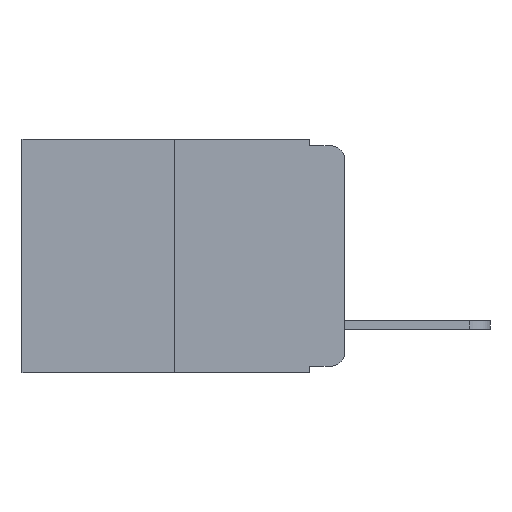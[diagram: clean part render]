
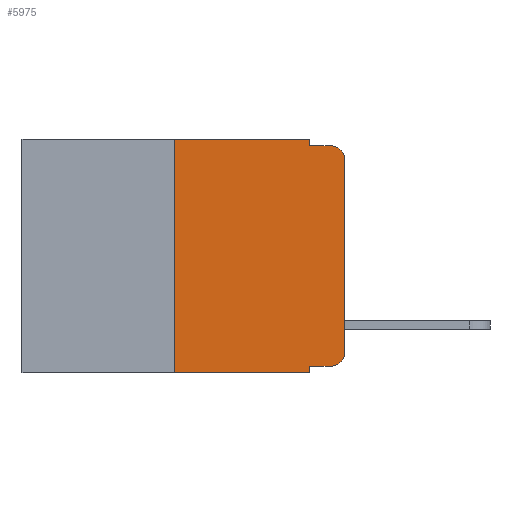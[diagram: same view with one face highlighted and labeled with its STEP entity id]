
A CAD part, left-side view. The second image highlights one B-rep face of the part: STEP entity #5975.
In plain terms, the highlighted planar face has unit normal (-1, 0, 0).
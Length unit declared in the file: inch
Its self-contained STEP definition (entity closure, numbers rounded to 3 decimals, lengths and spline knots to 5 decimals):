
#351 = CARTESIAN_POINT ( 'NONE',  ( 0., 0.473, 0. ) ) ;
#781 = CARTESIAN_POINT ( 'NONE',  ( 0., 0.051, 0. ) ) ;
#1145 = DIRECTION ( 'NONE',  ( 0., 0., -1. ) ) ;
#1237 = ORIENTED_EDGE ( 'NONE', *, *, #7425, .T. ) ;
#1449 = VERTEX_POINT ( 'NONE', #8383 ) ;
#1542 = CARTESIAN_POINT ( 'NONE',  ( 0., 0.02, -0.01 ) ) ;
#1710 = DIRECTION ( 'NONE',  ( 0., -1., 0. ) ) ;
#1713 = VERTEX_POINT ( 'NONE', #12270 ) ;
#1720 = DIRECTION ( 'NONE',  ( 0., 0., 1. ) ) ;
#1800 = FACE_OUTER_BOUND ( 'NONE', #14983, .T. ) ;
#2052 = LINE ( 'NONE', #19518, #5740 ) ;
#2232 = CARTESIAN_POINT ( 'NONE',  ( 0., 0.051, -0.333 ) ) ;
#2244 = EDGE_CURVE ( 'NONE', #5757, #9599, #10545, .T. ) ;
#2960 = VECTOR ( 'NONE', #1720, 39.37008 ) ;
#3056 = AXIS2_PLACEMENT_3D ( 'NONE', #4545, #17236, #6187 ) ;
#3840 = VERTEX_POINT ( 'NONE', #1542 ) ;
#3884 = VERTEX_POINT ( 'NONE', #6210 ) ;
#3897 = DIRECTION ( 'NONE',  ( 0., 0., -1. ) ) ;
#4142 = CARTESIAN_POINT ( 'NONE',  ( 0., 0.25, 0. ) ) ;
#4191 = ORIENTED_EDGE ( 'NONE', *, *, #17792, .F. ) ;
#4386 = ORIENTED_EDGE ( 'NONE', *, *, #19611, .T. ) ;
#4545 = CARTESIAN_POINT ( 'NONE',  ( 0., 0.02, -0.313 ) ) ;
#4651 = EDGE_CURVE ( 'NONE', #17564, #9599, #8992, .T. ) ;
#5457 = VERTEX_POINT ( 'NONE', #11801 ) ;
#5740 = VECTOR ( 'NONE', #13293, 39.37008 ) ;
#5757 = VERTEX_POINT ( 'NONE', #18464 ) ;
#5857 = VECTOR ( 'NONE', #1145, 39.37008 ) ;
#5975 = ADVANCED_FACE ( 'NONE', ( #1800 ), #18246, .F. ) ;
#5995 = CARTESIAN_POINT ( 'NONE',  ( 0., 0.051, 0. ) ) ;
#6005 = ORIENTED_EDGE ( 'NONE', *, *, #6626, .F. ) ;
#6187 = DIRECTION ( 'NONE',  ( 0., 0., -1. ) ) ;
#6210 = CARTESIAN_POINT ( 'NONE',  ( 0., 0., -0.313 ) ) ;
#6262 = DIRECTION ( 'NONE',  ( 0., -1., 0. ) ) ;
#6626 = EDGE_CURVE ( 'NONE', #5457, #3840, #11611, .T. ) ;
#6985 = DIRECTION ( 'NONE',  ( 0., 0., -1. ) ) ;
#7264 = EDGE_CURVE ( 'NONE', #12671, #3884, #17466, .T. ) ;
#7372 = ORIENTED_EDGE ( 'NONE', *, *, #4651, .T. ) ;
#7425 = EDGE_CURVE ( 'NONE', #3884, #1449, #9598, .T. ) ;
#7873 = CARTESIAN_POINT ( 'NONE',  ( 0., 0.051, -0.01 ) ) ;
#8383 = CARTESIAN_POINT ( 'NONE',  ( 0., 0., -0.03 ) ) ;
#8603 = DIRECTION ( 'NONE',  ( 0., -1., 0. ) ) ;
#8629 = VECTOR ( 'NONE', #8603, 39.37008 ) ;
#8707 = AXIS2_PLACEMENT_3D ( 'NONE', #19690, #8859, #3897 ) ;
#8859 = DIRECTION ( 'NONE',  ( 1., 0., 0. ) ) ;
#8992 = LINE ( 'NONE', #17459, #15130 ) ;
#9150 = EDGE_CURVE ( 'NONE', #5757, #12671, #10622, .T. ) ;
#9397 = ORIENTED_EDGE ( 'NONE', *, *, #13749, .F. ) ;
#9441 = DIRECTION ( 'NONE',  ( 0., -1., 0. ) ) ;
#9598 = LINE ( 'NONE', #12794, #2960 ) ;
#9599 = VERTEX_POINT ( 'NONE', #13038 ) ;
#10308 = VECTOR ( 'NONE', #1710, 39.37008 ) ;
#10396 = DIRECTION ( 'NONE',  ( 0., 0., 1. ) ) ;
#10545 = LINE ( 'NONE', #5995, #5857 ) ;
#10622 = LINE ( 'NONE', #2232, #8629 ) ;
#11278 = CARTESIAN_POINT ( 'NONE',  ( 0., 0.02, -0.03 ) ) ;
#11611 = LINE ( 'NONE', #7873, #18951 ) ;
#11801 = CARTESIAN_POINT ( 'NONE',  ( 0., 0.051, -0.01 ) ) ;
#12270 = CARTESIAN_POINT ( 'NONE',  ( 0., 0.25, 0. ) ) ;
#12671 = VERTEX_POINT ( 'NONE', #14905 ) ;
#12794 = CARTESIAN_POINT ( 'NONE',  ( 0., 0., 0. ) ) ;
#12839 = AXIS2_PLACEMENT_3D ( 'NONE', #11278, #12852, #6985 ) ;
#12852 = DIRECTION ( 'NONE',  ( -1., 0., 0. ) ) ;
#13038 = CARTESIAN_POINT ( 'NONE',  ( 0., 0.051, -0.343 ) ) ;
#13293 = DIRECTION ( 'NONE',  ( 0., 0., -1. ) ) ;
#13749 = EDGE_CURVE ( 'NONE', #17564, #1713, #19992, .T. ) ;
#14101 = ORIENTED_EDGE ( 'NONE', *, *, #9150, .T. ) ;
#14514 = ORIENTED_EDGE ( 'NONE', *, *, #19577, .F. ) ;
#14905 = CARTESIAN_POINT ( 'NONE',  ( 0., 0.02, -0.333 ) ) ;
#14983 = EDGE_LOOP ( 'NONE', ( #1237, #4386, #6005, #4191, #14514, #9397, #7372, #19859, #14101, #19854 ) ) ;
#15130 = VECTOR ( 'NONE', #6262, 39.37008 ) ;
#15465 = CIRCLE ( 'NONE', #12839, 0.02 ) ;
#15821 = VECTOR ( 'NONE', #10396, 39.37008 ) ;
#15950 = LINE ( 'NONE', #351, #10308 ) ;
#16530 = VERTEX_POINT ( 'NONE', #781 ) ;
#17236 = DIRECTION ( 'NONE',  ( -1., 0., 0. ) ) ;
#17269 = CARTESIAN_POINT ( 'NONE',  ( 0., 0.25, -0.343 ) ) ;
#17459 = CARTESIAN_POINT ( 'NONE',  ( 0., 0.473, -0.343 ) ) ;
#17466 = CIRCLE ( 'NONE', #3056, 0.02 ) ;
#17564 = VERTEX_POINT ( 'NONE', #17269 ) ;
#17792 = EDGE_CURVE ( 'NONE', #16530, #5457, #2052, .T. ) ;
#18246 = PLANE ( 'NONE',  #8707 ) ;
#18464 = CARTESIAN_POINT ( 'NONE',  ( 0., 0.051, -0.333 ) ) ;
#18951 = VECTOR ( 'NONE', #9441, 39.37008 ) ;
#19518 = CARTESIAN_POINT ( 'NONE',  ( 0., 0.051, 0. ) ) ;
#19577 = EDGE_CURVE ( 'NONE', #1713, #16530, #15950, .T. ) ;
#19611 = EDGE_CURVE ( 'NONE', #1449, #3840, #15465, .T. ) ;
#19690 = CARTESIAN_POINT ( 'NONE',  ( 0., 0.473, 0. ) ) ;
#19854 = ORIENTED_EDGE ( 'NONE', *, *, #7264, .T. ) ;
#19859 = ORIENTED_EDGE ( 'NONE', *, *, #2244, .F. ) ;
#19992 = LINE ( 'NONE', #4142, #15821 ) ;
